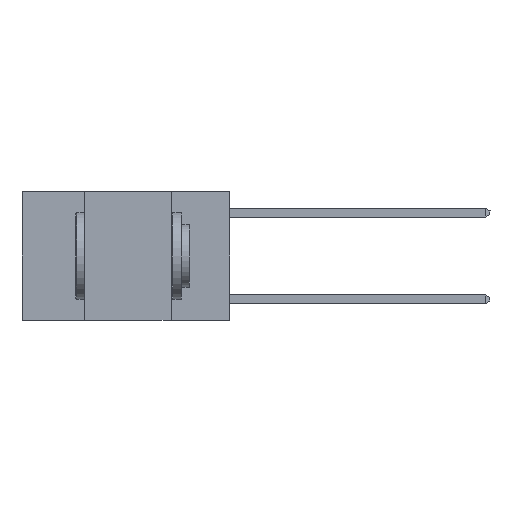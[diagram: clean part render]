
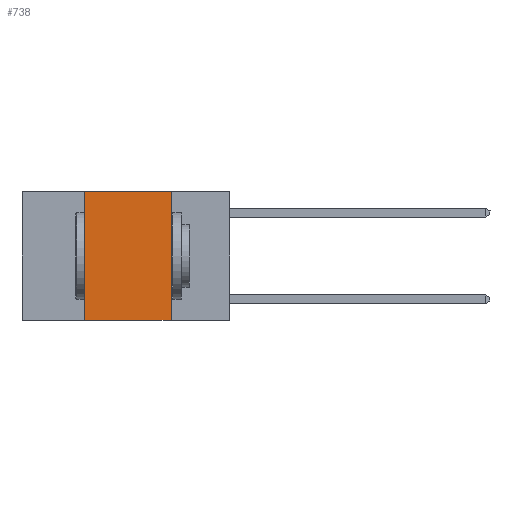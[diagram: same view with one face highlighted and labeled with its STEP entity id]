
A CAD part, left-side view. The second image highlights one B-rep face of the part: STEP entity #738.
In plain terms, the highlighted planar face has unit normal (-1, 0, 0).
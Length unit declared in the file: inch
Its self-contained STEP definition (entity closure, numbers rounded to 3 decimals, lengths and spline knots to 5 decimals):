
#400 = CARTESIAN_POINT ( 'NONE',  ( 0., 0.6, 0. ) ) ;
#738 = ADVANCED_FACE ( 'NONE', ( #4505 ), #19039, .F. ) ;
#1656 = VERTEX_POINT ( 'NONE', #14254 ) ;
#4448 = VERTEX_POINT ( 'NONE', #16777 ) ;
#4505 = FACE_OUTER_BOUND ( 'NONE', #20804, .T. ) ;
#4772 = LINE ( 'NONE', #5061, #24359 ) ;
#5061 = CARTESIAN_POINT ( 'NONE',  ( 0., 0.42, 0. ) ) ;
#5380 = EDGE_CURVE ( 'NONE', #1656, #17684, #4772, .T. ) ;
#6088 = CARTESIAN_POINT ( 'NONE',  ( 0., 0.17, 0. ) ) ;
#6174 = VERTEX_POINT ( 'NONE', #14800 ) ;
#6666 = EDGE_CURVE ( 'NONE', #1656, #4448, #8275, .T. ) ;
#7122 = VECTOR ( 'NONE', #9917, 39.37008 ) ;
#8275 = LINE ( 'NONE', #14281, #12713 ) ;
#8660 = DIRECTION ( 'NONE',  ( 0., -1., 0. ) ) ;
#8887 = DIRECTION ( 'NONE',  ( 0., 0., 1. ) ) ;
#8933 = ORIENTED_EDGE ( 'NONE', *, *, #5380, .F. ) ;
#9917 = DIRECTION ( 'NONE',  ( 0., 0., -1. ) ) ;
#11311 = DIRECTION ( 'NONE',  ( 0., -1., 0. ) ) ;
#12030 = DIRECTION ( 'NONE',  ( 1., 0., 0. ) ) ;
#12713 = VECTOR ( 'NONE', #8660, 39.37008 ) ;
#12767 = ORIENTED_EDGE ( 'NONE', *, *, #17171, .F. ) ;
#13945 = ORIENTED_EDGE ( 'NONE', *, *, #6666, .T. ) ;
#14254 = CARTESIAN_POINT ( 'NONE',  ( 0., 0.42, -0.37 ) ) ;
#14281 = CARTESIAN_POINT ( 'NONE',  ( 0., 0.6, -0.37 ) ) ;
#14800 = CARTESIAN_POINT ( 'NONE',  ( 0., 0.17, 0. ) ) ;
#16777 = CARTESIAN_POINT ( 'NONE',  ( 0., 0.17, -0.37 ) ) ;
#17094 = AXIS2_PLACEMENT_3D ( 'NONE', #400, #12030, #18840 ) ;
#17171 = EDGE_CURVE ( 'NONE', #6174, #4448, #17778, .T. ) ;
#17684 = VERTEX_POINT ( 'NONE', #24484 ) ;
#17691 = EDGE_CURVE ( 'NONE', #17684, #6174, #21667, .T. ) ;
#17778 = LINE ( 'NONE', #6088, #7122 ) ;
#17807 = ORIENTED_EDGE ( 'NONE', *, *, #17691, .F. ) ;
#18840 = DIRECTION ( 'NONE',  ( 0., 0., -1. ) ) ;
#19039 = PLANE ( 'NONE',  #17094 ) ;
#20442 = VECTOR ( 'NONE', #11311, 39.37008 ) ;
#20766 = CARTESIAN_POINT ( 'NONE',  ( 0., 0.6, 0. ) ) ;
#20804 = EDGE_LOOP ( 'NONE', ( #12767, #17807, #8933, #13945 ) ) ;
#21667 = LINE ( 'NONE', #20766, #20442 ) ;
#24359 = VECTOR ( 'NONE', #8887, 39.37008 ) ;
#24484 = CARTESIAN_POINT ( 'NONE',  ( 0., 0.42, 0. ) ) ;
